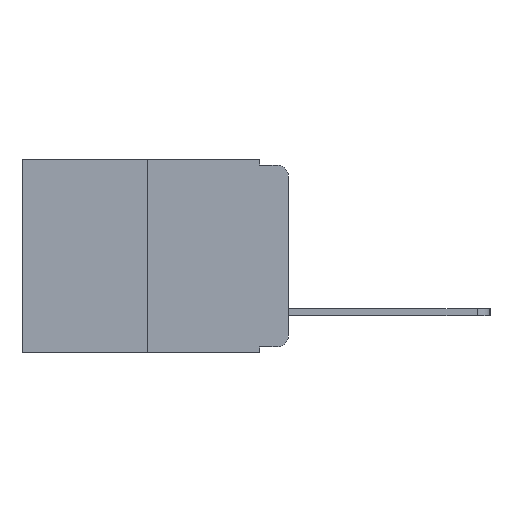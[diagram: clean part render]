
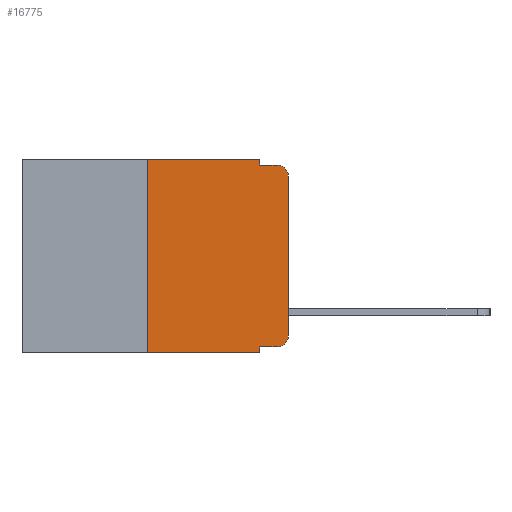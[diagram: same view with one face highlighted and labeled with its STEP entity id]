
A CAD part, left-side view. The second image highlights one B-rep face of the part: STEP entity #16775.
In plain terms, the highlighted planar face has unit normal (-1, 0, 0).
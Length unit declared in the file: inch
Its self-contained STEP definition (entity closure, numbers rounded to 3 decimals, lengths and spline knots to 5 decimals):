
#132 = VERTEX_POINT ( 'NONE', #15179 ) ;
#511 = EDGE_CURVE ( 'NONE', #16547, #18840, #18922, .T. ) ;
#687 = ORIENTED_EDGE ( 'NONE', *, *, #7902, .T. ) ;
#856 = CARTESIAN_POINT ( 'NONE',  ( 0., 0.051, -0.333 ) ) ;
#857 = VECTOR ( 'NONE', #4706, 39.37008 ) ;
#864 = DIRECTION ( 'NONE',  ( 0., 0., -1. ) ) ;
#1069 = EDGE_CURVE ( 'NONE', #11777, #19392, #9195, .T. ) ;
#1552 = VERTEX_POINT ( 'NONE', #9619 ) ;
#1653 = VECTOR ( 'NONE', #3882, 39.37008 ) ;
#1787 = ORIENTED_EDGE ( 'NONE', *, *, #4724, .T. ) ;
#2318 = VECTOR ( 'NONE', #18280, 39.37008 ) ;
#2462 = VECTOR ( 'NONE', #7916, 39.37008 ) ;
#2550 = DIRECTION ( 'NONE',  ( 0., -1., 0. ) ) ;
#2659 = VERTEX_POINT ( 'NONE', #856 ) ;
#3036 = CARTESIAN_POINT ( 'NONE',  ( 0., 0.25, 0. ) ) ;
#3275 = CARTESIAN_POINT ( 'NONE',  ( 0., 0.473, -0.343 ) ) ;
#3664 = VERTEX_POINT ( 'NONE', #11828 ) ;
#3882 = DIRECTION ( 'NONE',  ( 0., -1., 0. ) ) ;
#4059 = CARTESIAN_POINT ( 'NONE',  ( 0., 0.02, -0.01 ) ) ;
#4686 = ORIENTED_EDGE ( 'NONE', *, *, #10970, .F. ) ;
#4706 = DIRECTION ( 'NONE',  ( 0., 0., 1. ) ) ;
#4724 = EDGE_CURVE ( 'NONE', #1552, #3664, #6819, .T. ) ;
#4901 = ORIENTED_EDGE ( 'NONE', *, *, #1069, .T. ) ;
#5750 = VERTEX_POINT ( 'NONE', #8924 ) ;
#5753 = EDGE_CURVE ( 'NONE', #132, #9912, #18306, .T. ) ;
#5769 = PLANE ( 'NONE',  #11212 ) ;
#5989 = FACE_OUTER_BOUND ( 'NONE', #17952, .T. ) ;
#6398 = ORIENTED_EDGE ( 'NONE', *, *, #13929, .F. ) ;
#6640 = DIRECTION ( 'NONE',  ( -1., 0., 0. ) ) ;
#6819 = CIRCLE ( 'NONE', #15636, 0.02 ) ;
#7149 = DIRECTION ( 'NONE',  ( 0., 0., -1. ) ) ;
#7370 = DIRECTION ( 'NONE',  ( 0., -1., 0. ) ) ;
#7581 = AXIS2_PLACEMENT_3D ( 'NONE', #9433, #6640, #7149 ) ;
#7666 = EDGE_CURVE ( 'NONE', #3664, #11777, #18263, .T. ) ;
#7745 = VECTOR ( 'NONE', #8115, 39.37008 ) ;
#7902 = EDGE_CURVE ( 'NONE', #2659, #1552, #14086, .T. ) ;
#7916 = DIRECTION ( 'NONE',  ( 0., 0., 1. ) ) ;
#8056 = CARTESIAN_POINT ( 'NONE',  ( 0., 0.051, 0. ) ) ;
#8115 = DIRECTION ( 'NONE',  ( 0., 0., -1. ) ) ;
#8574 = ORIENTED_EDGE ( 'NONE', *, *, #5753, .F. ) ;
#8924 = CARTESIAN_POINT ( 'NONE',  ( 0., 0.051, -0.01 ) ) ;
#9051 = CARTESIAN_POINT ( 'NONE',  ( 0., 0.051, -0.343 ) ) ;
#9082 = ORIENTED_EDGE ( 'NONE', *, *, #7666, .T. ) ;
#9195 = CIRCLE ( 'NONE', #7581, 0.02 ) ;
#9348 = CARTESIAN_POINT ( 'NONE',  ( 0., 0.051, 0. ) ) ;
#9433 = CARTESIAN_POINT ( 'NONE',  ( 0., 0.02, -0.03 ) ) ;
#9568 = ORIENTED_EDGE ( 'NONE', *, *, #511, .T. ) ;
#9619 = CARTESIAN_POINT ( 'NONE',  ( 0., 0.02, -0.333 ) ) ;
#9912 = VERTEX_POINT ( 'NONE', #9348 ) ;
#10469 = VECTOR ( 'NONE', #7370, 39.37008 ) ;
#10487 = DIRECTION ( 'NONE',  ( 1., 0., 0. ) ) ;
#10970 = EDGE_CURVE ( 'NONE', #2659, #18840, #18130, .T. ) ;
#11212 = AXIS2_PLACEMENT_3D ( 'NONE', #19289, #10487, #864 ) ;
#11468 = CARTESIAN_POINT ( 'NONE',  ( 0., 0.25, -0.343 ) ) ;
#11620 = CARTESIAN_POINT ( 'NONE',  ( 0., 0.051, -0.333 ) ) ;
#11777 = VERTEX_POINT ( 'NONE', #13694 ) ;
#11828 = CARTESIAN_POINT ( 'NONE',  ( 0., 0., -0.313 ) ) ;
#12025 = CARTESIAN_POINT ( 'NONE',  ( 0., 0.051, -0.01 ) ) ;
#12117 = EDGE_CURVE ( 'NONE', #5750, #19392, #17578, .T. ) ;
#12144 = DIRECTION ( 'NONE',  ( -1., 0., 0. ) ) ;
#12203 = CARTESIAN_POINT ( 'NONE',  ( 0., 0.02, -0.313 ) ) ;
#12973 = EDGE_CURVE ( 'NONE', #16547, #132, #13442, .T. ) ;
#13442 = LINE ( 'NONE', #3036, #857 ) ;
#13666 = VECTOR ( 'NONE', #2550, 39.37008 ) ;
#13694 = CARTESIAN_POINT ( 'NONE',  ( 0., 0., -0.03 ) ) ;
#13929 = EDGE_CURVE ( 'NONE', #9912, #5750, #15684, .T. ) ;
#14086 = LINE ( 'NONE', #11620, #1653 ) ;
#15025 = VECTOR ( 'NONE', #19758, 39.37008 ) ;
#15179 = CARTESIAN_POINT ( 'NONE',  ( 0., 0.25, 0. ) ) ;
#15636 = AXIS2_PLACEMENT_3D ( 'NONE', #12203, #12144, #17903 ) ;
#15684 = LINE ( 'NONE', #8056, #7745 ) ;
#16547 = VERTEX_POINT ( 'NONE', #11468 ) ;
#16775 = ADVANCED_FACE ( 'NONE', ( #5989 ), #5769, .F. ) ;
#16813 = CARTESIAN_POINT ( 'NONE',  ( 0., 0.051, 0. ) ) ;
#16932 = CARTESIAN_POINT ( 'NONE',  ( 0., 0., 0. ) ) ;
#17578 = LINE ( 'NONE', #12025, #13666 ) ;
#17873 = CARTESIAN_POINT ( 'NONE',  ( 0., 0.473, 0. ) ) ;
#17903 = DIRECTION ( 'NONE',  ( 0., 0., -1. ) ) ;
#17952 = EDGE_LOOP ( 'NONE', ( #9082, #4901, #19456, #6398, #8574, #19893, #9568, #4686, #687, #1787 ) ) ;
#18130 = LINE ( 'NONE', #16813, #2318 ) ;
#18263 = LINE ( 'NONE', #16932, #2462 ) ;
#18280 = DIRECTION ( 'NONE',  ( 0., 0., -1. ) ) ;
#18306 = LINE ( 'NONE', #17873, #10469 ) ;
#18840 = VERTEX_POINT ( 'NONE', #9051 ) ;
#18922 = LINE ( 'NONE', #3275, #15025 ) ;
#19289 = CARTESIAN_POINT ( 'NONE',  ( 0., 0.473, 0. ) ) ;
#19392 = VERTEX_POINT ( 'NONE', #4059 ) ;
#19456 = ORIENTED_EDGE ( 'NONE', *, *, #12117, .F. ) ;
#19758 = DIRECTION ( 'NONE',  ( 0., -1., 0. ) ) ;
#19893 = ORIENTED_EDGE ( 'NONE', *, *, #12973, .F. ) ;
